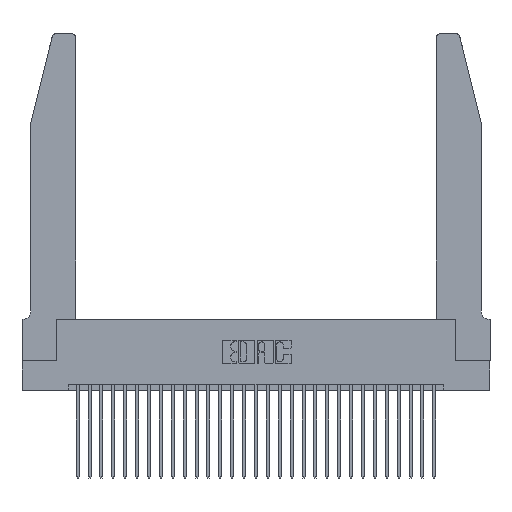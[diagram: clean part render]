
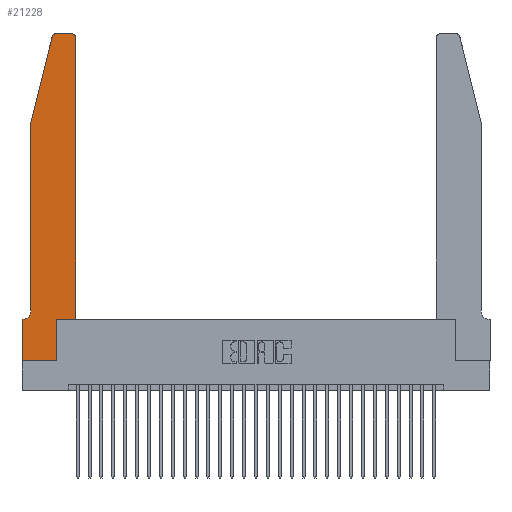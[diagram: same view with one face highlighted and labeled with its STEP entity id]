
A CAD part, top view. The second image highlights one B-rep face of the part: STEP entity #21228.
In plain terms, the highlighted planar face has unit normal (0, 0, 1).
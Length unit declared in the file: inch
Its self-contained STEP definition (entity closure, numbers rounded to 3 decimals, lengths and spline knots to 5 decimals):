
#53 = EDGE_LOOP ( 'NONE', ( #22434, #11567, #28781, #26205, #23657, #30494, #15042, #19732, #2608, #8614, #8559, #22683 ) ) ;
#395 = CARTESIAN_POINT ( 'NONE',  ( 0., 0., 0.37 ) ) ;
#693 = CARTESIAN_POINT ( 'NONE',  ( 0., 0.35, 0.37 ) ) ;
#974 = DIRECTION ( 'NONE',  ( 0., 0., 1. ) ) ;
#1277 = CARTESIAN_POINT ( 'NONE',  ( 0.0755, 2., 0.37 ) ) ;
#1528 = CARTESIAN_POINT ( 'NONE',  ( 0.2865, 0.35, 0.37 ) ) ;
#1743 = CARTESIAN_POINT ( 'NONE',  ( 0.25487, 2.72718, 0.37 ) ) ;
#1989 = VERTEX_POINT ( 'NONE', #29692 ) ;
#2111 = DIRECTION ( 'NONE',  ( 0., -1., 0. ) ) ;
#2608 = ORIENTED_EDGE ( 'NONE', *, *, #2958, .T. ) ;
#2952 = FACE_OUTER_BOUND ( 'NONE', #53, .T. ) ;
#2958 = EDGE_CURVE ( 'NONE', #10972, #10611, #16801, .T. ) ;
#3080 = CIRCLE ( 'NONE', #12558, 0.03 ) ;
#3138 = DIRECTION ( 'NONE',  ( 0., -1., 0. ) ) ;
#3279 = CARTESIAN_POINT ( 'NONE',  ( 0.0055, 0.35, 0.37 ) ) ;
#3509 = DIRECTION ( 'NONE',  ( 1., 0., 0. ) ) ;
#4284 = VECTOR ( 'NONE', #23775, 39.37008 ) ;
#4858 = CARTESIAN_POINT ( 'NONE',  ( 0.2865, 0.35, 0.37 ) ) ;
#5155 = VERTEX_POINT ( 'NONE', #23553 ) ;
#5168 = VECTOR ( 'NONE', #2111, 39.37008 ) ;
#5295 = VECTOR ( 'NONE', #6057, 39.37008 ) ;
#6057 = DIRECTION ( 'NONE',  ( -0.239, -0.971, 0. ) ) ;
#6479 = LINE ( 'NONE', #21727, #4284 ) ;
#6643 = CARTESIAN_POINT ( 'NONE',  ( 0., 0., 0.37 ) ) ;
#7192 = VECTOR ( 'NONE', #3138, 39.37008 ) ;
#7870 = EDGE_CURVE ( 'NONE', #11477, #13327, #20531, .T. ) ;
#8559 = ORIENTED_EDGE ( 'NONE', *, *, #7870, .T. ) ;
#8590 = VERTEX_POINT ( 'NONE', #1743 ) ;
#8614 = ORIENTED_EDGE ( 'NONE', *, *, #21587, .T. ) ;
#8933 = EDGE_CURVE ( 'NONE', #8590, #23384, #22644, .T. ) ;
#9517 = VECTOR ( 'NONE', #26334, 39.37008 ) ;
#9569 = DIRECTION ( 'NONE',  ( 0., 1., 0. ) ) ;
#10611 = VERTEX_POINT ( 'NONE', #1528 ) ;
#10972 = VERTEX_POINT ( 'NONE', #17370 ) ;
#11008 = VERTEX_POINT ( 'NONE', #693 ) ;
#11477 = VERTEX_POINT ( 'NONE', #24128 ) ;
#11567 = ORIENTED_EDGE ( 'NONE', *, *, #21498, .T. ) ;
#12558 = AXIS2_PLACEMENT_3D ( 'NONE', #20216, #974, #3509 ) ;
#12574 = DIRECTION ( 'NONE',  ( 0., 0., -1. ) ) ;
#13107 = LINE ( 'NONE', #16981, #7192 ) ;
#13327 = VERTEX_POINT ( 'NONE', #27201 ) ;
#13762 = CARTESIAN_POINT ( 'NONE',  ( 0., 0., 0.37 ) ) ;
#14289 = VERTEX_POINT ( 'NONE', #3279 ) ;
#14527 = LINE ( 'NONE', #13762, #21527 ) ;
#15042 = ORIENTED_EDGE ( 'NONE', *, *, #17781, .T. ) ;
#15164 = EDGE_CURVE ( 'NONE', #23384, #5155, #13107, .T. ) ;
#15367 = VECTOR ( 'NONE', #16095, 39.37008 ) ;
#15812 = DIRECTION ( 'NONE',  ( 0., 0., 1. ) ) ;
#15988 = DIRECTION ( 'NONE',  ( 1., 0., 0. ) ) ;
#16095 = DIRECTION ( 'NONE',  ( 0., 1., 0. ) ) ;
#16177 = EDGE_CURVE ( 'NONE', #5155, #14289, #21185, .T. ) ;
#16801 = LINE ( 'NONE', #4858, #17531 ) ;
#16846 = VERTEX_POINT ( 'NONE', #395 ) ;
#16981 = CARTESIAN_POINT ( 'NONE',  ( 0.0755, 2., 0.37 ) ) ;
#17327 = VECTOR ( 'NONE', #15988, 39.37008 ) ;
#17370 = CARTESIAN_POINT ( 'NONE',  ( 0.2865, 0., 0.37 ) ) ;
#17531 = VECTOR ( 'NONE', #9569, 39.37008 ) ;
#17781 = EDGE_CURVE ( 'NONE', #11008, #16846, #19961, .T. ) ;
#18347 = VERTEX_POINT ( 'NONE', #20981 ) ;
#18611 = DIRECTION ( 'NONE',  ( 1., 0., 0. ) ) ;
#19146 = DIRECTION ( 'NONE',  ( 0., 0., 1. ) ) ;
#19732 = ORIENTED_EDGE ( 'NONE', *, *, #27988, .T. ) ;
#19938 = EDGE_CURVE ( 'NONE', #18347, #1989, #27961, .T. ) ;
#19961 = LINE ( 'NONE', #6643, #5168 ) ;
#20098 = AXIS2_PLACEMENT_3D ( 'NONE', #26236, #12574, #22754 ) ;
#20216 = CARTESIAN_POINT ( 'NONE',  ( 0.4205, 2.72, 0.37 ) ) ;
#20330 = DIRECTION ( 'NONE',  ( 1., 0., 0. ) ) ;
#20531 = LINE ( 'NONE', #21026, #15367 ) ;
#20981 = CARTESIAN_POINT ( 'NONE',  ( 0.4205, 2.75, 0.37 ) ) ;
#21026 = CARTESIAN_POINT ( 'NONE',  ( 0.4505, 0.35, 0.37 ) ) ;
#21185 = CIRCLE ( 'NONE', #20098, 0.07 ) ;
#21228 = ADVANCED_FACE ( 'NONE', ( #2952 ), #29920, .T. ) ;
#21498 = EDGE_CURVE ( 'NONE', #1989, #8590, #25443, .T. ) ;
#21518 = DIRECTION ( 'NONE',  ( 1., 0., 0. ) ) ;
#21527 = VECTOR ( 'NONE', #20330, 39.37008 ) ;
#21587 = EDGE_CURVE ( 'NONE', #10611, #11477, #28741, .T. ) ;
#21727 = CARTESIAN_POINT ( 'NONE',  ( 0.0755, 0.35, 0.37 ) ) ;
#22434 = ORIENTED_EDGE ( 'NONE', *, *, #19938, .T. ) ;
#22644 = LINE ( 'NONE', #1277, #5295 ) ;
#22683 = ORIENTED_EDGE ( 'NONE', *, *, #25245, .T. ) ;
#22754 = DIRECTION ( 'NONE',  ( -1., 0., 0. ) ) ;
#22784 = CARTESIAN_POINT ( 'NONE',  ( 0., 0.35, 0.37 ) ) ;
#23334 = AXIS2_PLACEMENT_3D ( 'NONE', #28500, #19146, #21518 ) ;
#23384 = VERTEX_POINT ( 'NONE', #28310 ) ;
#23553 = CARTESIAN_POINT ( 'NONE',  ( 0.0755, 0.42, 0.37 ) ) ;
#23566 = EDGE_CURVE ( 'NONE', #14289, #11008, #6479, .T. ) ;
#23657 = ORIENTED_EDGE ( 'NONE', *, *, #16177, .T. ) ;
#23775 = DIRECTION ( 'NONE',  ( -1., 0., 0. ) ) ;
#24128 = CARTESIAN_POINT ( 'NONE',  ( 0.4505, 0.35, 0.37 ) ) ;
#25245 = EDGE_CURVE ( 'NONE', #13327, #18347, #3080, .T. ) ;
#25443 = CIRCLE ( 'NONE', #23334, 0.03 ) ;
#26205 = ORIENTED_EDGE ( 'NONE', *, *, #15164, .T. ) ;
#26236 = CARTESIAN_POINT ( 'NONE',  ( 0.0055, 0.42, 0.37 ) ) ;
#26334 = DIRECTION ( 'NONE',  ( -1., 0., 0. ) ) ;
#26530 = CARTESIAN_POINT ( 'NONE',  ( 0.2605, 2.75, 0.37 ) ) ;
#27201 = CARTESIAN_POINT ( 'NONE',  ( 0.4505, 2.72, 0.37 ) ) ;
#27900 = CARTESIAN_POINT ( 'NONE',  ( 0.4505, 0.35, 0.37 ) ) ;
#27961 = LINE ( 'NONE', #26530, #9517 ) ;
#27988 = EDGE_CURVE ( 'NONE', #16846, #10972, #14527, .T. ) ;
#28310 = CARTESIAN_POINT ( 'NONE',  ( 0.0755, 2., 0.37 ) ) ;
#28500 = CARTESIAN_POINT ( 'NONE',  ( 0.284, 2.72, 0.37 ) ) ;
#28741 = LINE ( 'NONE', #27900, #17327 ) ;
#28781 = ORIENTED_EDGE ( 'NONE', *, *, #8933, .T. ) ;
#29692 = CARTESIAN_POINT ( 'NONE',  ( 0.284, 2.75, 0.37 ) ) ;
#29920 = PLANE ( 'NONE',  #30260 ) ;
#30260 = AXIS2_PLACEMENT_3D ( 'NONE', #22784, #15812, #18611 ) ;
#30494 = ORIENTED_EDGE ( 'NONE', *, *, #23566, .T. ) ;
